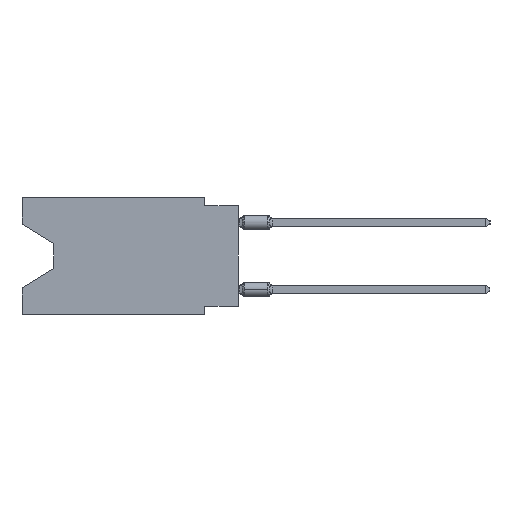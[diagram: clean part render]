
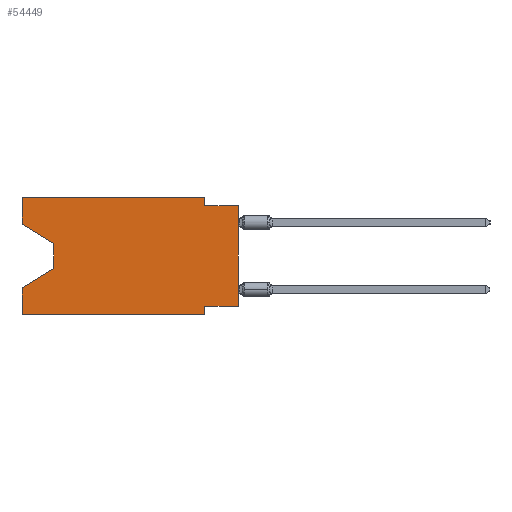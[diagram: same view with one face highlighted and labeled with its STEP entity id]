
A CAD part, left-side view. The second image highlights one B-rep face of the part: STEP entity #54449.
In plain terms, the highlighted planar face has unit normal (-1, 0, 0).
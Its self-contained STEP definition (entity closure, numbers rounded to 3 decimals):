
#433 = EDGE_LOOP ( 'NONE', ( #31181, #10536, #18421, #11688, #43213, #50227, #24711, #11035, #30085, #32580, #3926, #35978 ) ) ;
#916 = VERTEX_POINT ( 'NONE', #49754 ) ;
#1885 = DIRECTION ( 'NONE',  ( 0., 0., -1. ) ) ;
#3134 = CARTESIAN_POINT ( 'NONE',  ( 0., 0., 0. ) ) ;
#3489 = VECTOR ( 'NONE', #38751, 1000. ) ;
#3926 = ORIENTED_EDGE ( 'NONE', *, *, #34598, .F. ) ;
#4495 = EDGE_CURVE ( 'NONE', #20165, #32952, #19424, .T. ) ;
#7393 = VECTOR ( 'NONE', #35912, 1000. ) ;
#8024 = LINE ( 'NONE', #33776, #3489 ) ;
#8260 = DIRECTION ( 'NONE',  ( 0., 0., 1. ) ) ;
#10499 = CARTESIAN_POINT ( 'NONE',  ( 0., 16.383, 0. ) ) ;
#10536 = ORIENTED_EDGE ( 'NONE', *, *, #33820, .T. ) ;
#10596 = CARTESIAN_POINT ( 'NONE',  ( 0., 2.54, 0. ) ) ;
#10725 = DIRECTION ( 'NONE',  ( 1., 0., 0. ) ) ;
#11035 = ORIENTED_EDGE ( 'NONE', *, *, #4495, .T. ) ;
#11688 = ORIENTED_EDGE ( 'NONE', *, *, #20283, .F. ) ;
#12361 = CARTESIAN_POINT ( 'NONE',  ( 0., 16.383, -2.038 ) ) ;
#12952 = CARTESIAN_POINT ( 'NONE',  ( 0., 16.383, 0. ) ) ;
#13034 = EDGE_CURVE ( 'NONE', #50446, #29702, #8024, .T. ) ;
#13469 = VERTEX_POINT ( 'NONE', #42776 ) ;
#14610 = PLANE ( 'NONE',  #34542 ) ;
#14917 = DIRECTION ( 'NONE',  ( 0., -1., 0. ) ) ;
#16169 = LINE ( 'NONE', #50192, #17949 ) ;
#17119 = LINE ( 'NONE', #12952, #52136 ) ;
#17239 = VECTOR ( 'NONE', #21999, 1000. ) ;
#17949 = VECTOR ( 'NONE', #33055, 1000. ) ;
#18421 = ORIENTED_EDGE ( 'NONE', *, *, #24338, .T. ) ;
#18519 = DIRECTION ( 'NONE',  ( 0., -1., 0. ) ) ;
#18710 = VECTOR ( 'NONE', #18792, 1000. ) ;
#18792 = DIRECTION ( 'NONE',  ( 0., 1., 0. ) ) ;
#19018 = CARTESIAN_POINT ( 'NONE',  ( 0., 16.383, -2.038 ) ) ;
#19305 = EDGE_CURVE ( 'NONE', #20165, #13469, #22939, .T. ) ;
#19368 = CARTESIAN_POINT ( 'NONE',  ( 0., 13.97, -5.385 ) ) ;
#19424 = LINE ( 'NONE', #3134, #25798 ) ;
#19520 = VERTEX_POINT ( 'NONE', #31724 ) ;
#19607 = VERTEX_POINT ( 'NONE', #49985 ) ;
#20165 = VERTEX_POINT ( 'NONE', #34951 ) ;
#20283 = EDGE_CURVE ( 'NONE', #32827, #38867, #25536, .T. ) ;
#20805 = EDGE_CURVE ( 'NONE', #24519, #19607, #23182, .T. ) ;
#20836 = CARTESIAN_POINT ( 'NONE',  ( 0., 13.97, -5.385 ) ) ;
#21397 = CARTESIAN_POINT ( 'NONE',  ( 0., 16.383, 0. ) ) ;
#21999 = DIRECTION ( 'NONE',  ( 0., 0., -1. ) ) ;
#22152 = LINE ( 'NONE', #10499, #24021 ) ;
#22370 = VECTOR ( 'NONE', #34132, 1000. ) ;
#22828 = DIRECTION ( 'NONE',  ( 0., 0., -1. ) ) ;
#22939 = LINE ( 'NONE', #53114, #18710 ) ;
#23182 = LINE ( 'NONE', #19018, #7393 ) ;
#24021 = VECTOR ( 'NONE', #18519, 1000. ) ;
#24338 = EDGE_CURVE ( 'NONE', #27092, #38867, #52346, .T. ) ;
#24519 = VERTEX_POINT ( 'NONE', #12361 ) ;
#24681 = VECTOR ( 'NONE', #43484, 1000. ) ;
#24711 = ORIENTED_EDGE ( 'NONE', *, *, #19305, .F. ) ;
#25536 = LINE ( 'NONE', #21397, #22370 ) ;
#25798 = VECTOR ( 'NONE', #40482, 1000. ) ;
#27092 = VERTEX_POINT ( 'NONE', #20836 ) ;
#29219 = VECTOR ( 'NONE', #22828, 1000. ) ;
#29702 = VERTEX_POINT ( 'NONE', #50731 ) ;
#30085 = ORIENTED_EDGE ( 'NONE', *, *, #47037, .F. ) ;
#30611 = CARTESIAN_POINT ( 'NONE',  ( 0., 2.54, -8.89 ) ) ;
#30847 = LINE ( 'NONE', #30611, #17239 ) ;
#31181 = ORIENTED_EDGE ( 'NONE', *, *, #20805, .T. ) ;
#31651 = EDGE_CURVE ( 'NONE', #24519, #19520, #17119, .T. ) ;
#31724 = CARTESIAN_POINT ( 'NONE',  ( 0., 16.383, 0. ) ) ;
#31754 = CARTESIAN_POINT ( 'NONE',  ( 0., 16.383, 0. ) ) ;
#32580 = ORIENTED_EDGE ( 'NONE', *, *, #13034, .F. ) ;
#32827 = VERTEX_POINT ( 'NONE', #33197 ) ;
#32952 = VERTEX_POINT ( 'NONE', #46714 ) ;
#33055 = DIRECTION ( 'NONE',  ( 0., -1., 0. ) ) ;
#33197 = CARTESIAN_POINT ( 'NONE',  ( 0., 16.383, -8.89 ) ) ;
#33776 = CARTESIAN_POINT ( 'NONE',  ( 0., 2.54, 0. ) ) ;
#33820 = EDGE_CURVE ( 'NONE', #19607, #27092, #44121, .T. ) ;
#34132 = DIRECTION ( 'NONE',  ( 0., 0., 1. ) ) ;
#34542 = AXIS2_PLACEMENT_3D ( 'NONE', #31754, #10725, #1885 ) ;
#34598 = EDGE_CURVE ( 'NONE', #19520, #50446, #22152, .T. ) ;
#34951 = CARTESIAN_POINT ( 'NONE',  ( 0., 0., -8.255 ) ) ;
#35708 = CARTESIAN_POINT ( 'NONE',  ( 0., 0., -0.635 ) ) ;
#35912 = DIRECTION ( 'NONE',  ( 0., -0.855, -0.519 ) ) ;
#35978 = ORIENTED_EDGE ( 'NONE', *, *, #31651, .F. ) ;
#38652 = EDGE_CURVE ( 'NONE', #32827, #916, #16169, .T. ) ;
#38751 = DIRECTION ( 'NONE',  ( 0., 0., -1. ) ) ;
#38867 = VERTEX_POINT ( 'NONE', #48489 ) ;
#39789 = FACE_OUTER_BOUND ( 'NONE', #433, .T. ) ;
#39839 = LINE ( 'NONE', #35708, #44632 ) ;
#40482 = DIRECTION ( 'NONE',  ( 0., 0., 1. ) ) ;
#42776 = CARTESIAN_POINT ( 'NONE',  ( 0., 2.54, -8.255 ) ) ;
#43213 = ORIENTED_EDGE ( 'NONE', *, *, #38652, .T. ) ;
#43484 = DIRECTION ( 'NONE',  ( 0., 0.855, -0.519 ) ) ;
#44121 = LINE ( 'NONE', #52737, #29219 ) ;
#44632 = VECTOR ( 'NONE', #14917, 1000. ) ;
#46714 = CARTESIAN_POINT ( 'NONE',  ( 0., 0., -0.635 ) ) ;
#47037 = EDGE_CURVE ( 'NONE', #29702, #32952, #39839, .T. ) ;
#47383 = EDGE_CURVE ( 'NONE', #13469, #916, #30847, .T. ) ;
#48489 = CARTESIAN_POINT ( 'NONE',  ( 0., 16.383, -6.852 ) ) ;
#49754 = CARTESIAN_POINT ( 'NONE',  ( 0., 2.54, -8.89 ) ) ;
#49985 = CARTESIAN_POINT ( 'NONE',  ( 0., 13.97, -3.505 ) ) ;
#50192 = CARTESIAN_POINT ( 'NONE',  ( 0., 16.383, -8.89 ) ) ;
#50227 = ORIENTED_EDGE ( 'NONE', *, *, #47383, .F. ) ;
#50446 = VERTEX_POINT ( 'NONE', #10596 ) ;
#50731 = CARTESIAN_POINT ( 'NONE',  ( 0., 2.54, -0.635 ) ) ;
#52136 = VECTOR ( 'NONE', #8260, 1000. ) ;
#52346 = LINE ( 'NONE', #19368, #24681 ) ;
#52737 = CARTESIAN_POINT ( 'NONE',  ( 0., 13.97, -3.505 ) ) ;
#53114 = CARTESIAN_POINT ( 'NONE',  ( 0., 0., -8.255 ) ) ;
#54449 = ADVANCED_FACE ( 'NONE', ( #39789 ), #14610, .F. ) ;
